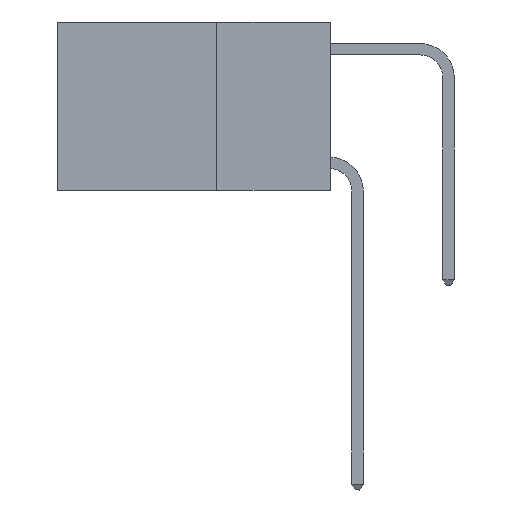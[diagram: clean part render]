
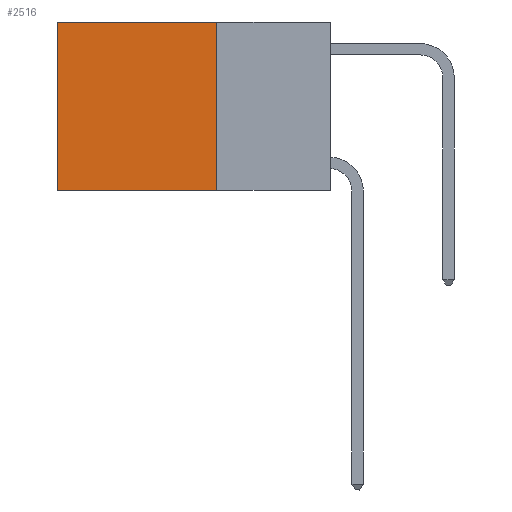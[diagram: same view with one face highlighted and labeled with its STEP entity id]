
A CAD part, left-side view. The second image highlights one B-rep face of the part: STEP entity #2516.
In plain terms, the highlighted planar face has unit normal (-1, 0, 0).
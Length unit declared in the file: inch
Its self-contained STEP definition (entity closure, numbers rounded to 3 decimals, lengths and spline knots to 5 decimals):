
#1464 = VECTOR ( 'NONE', #6346, 39.37008 ) ;
#2185 = ORIENTED_EDGE ( 'NONE', *, *, #26075, .F. ) ;
#2516 = ADVANCED_FACE ( 'NONE', ( #10999 ), #21430, .F. ) ;
#2658 = CARTESIAN_POINT ( 'NONE',  ( 0.2625, 0.25, 0. ) ) ;
#2849 = VERTEX_POINT ( 'NONE', #7916 ) ;
#4183 = LINE ( 'NONE', #4329, #1464 ) ;
#4329 = CARTESIAN_POINT ( 'NONE',  ( 0.2625, 0.25, -0.37 ) ) ;
#4627 = DIRECTION ( 'NONE',  ( 0., 0., -1. ) ) ;
#6046 = DIRECTION ( 'NONE',  ( 1., 0., 0. ) ) ;
#6346 = DIRECTION ( 'NONE',  ( 0., 1., 0. ) ) ;
#7273 = DIRECTION ( 'NONE',  ( 0., 0., -1. ) ) ;
#7916 = CARTESIAN_POINT ( 'NONE',  ( 0.2625, 0.6, -0.37 ) ) ;
#8099 = DIRECTION ( 'NONE',  ( 0., 0., -1. ) ) ;
#9724 = CARTESIAN_POINT ( 'NONE',  ( 0.2625, 0.6, 0. ) ) ;
#10724 = LINE ( 'NONE', #15518, #16401 ) ;
#10946 = CARTESIAN_POINT ( 'NONE',  ( 0.2625, 0.25, 0. ) ) ;
#10999 = FACE_OUTER_BOUND ( 'NONE', #18602, .T. ) ;
#11316 = ORIENTED_EDGE ( 'NONE', *, *, #17444, .T. ) ;
#15248 = ORIENTED_EDGE ( 'NONE', *, *, #21425, .F. ) ;
#15518 = CARTESIAN_POINT ( 'NONE',  ( 0.2625, 0.25, 0. ) ) ;
#16019 = EDGE_CURVE ( 'NONE', #23836, #22442, #22501, .T. ) ;
#16401 = VECTOR ( 'NONE', #4627, 39.37008 ) ;
#17006 = AXIS2_PLACEMENT_3D ( 'NONE', #19843, #6046, #8099 ) ;
#17444 = EDGE_CURVE ( 'NONE', #22442, #2849, #25091, .T. ) ;
#18409 = ORIENTED_EDGE ( 'NONE', *, *, #16019, .T. ) ;
#18602 = EDGE_LOOP ( 'NONE', ( #11316, #15248, #2185, #18409 ) ) ;
#18918 = VERTEX_POINT ( 'NONE', #27171 ) ;
#19843 = CARTESIAN_POINT ( 'NONE',  ( 0.2625, 0.25, 0. ) ) ;
#20331 = DIRECTION ( 'NONE',  ( 0., 1., 0. ) ) ;
#21425 = EDGE_CURVE ( 'NONE', #18918, #2849, #4183, .T. ) ;
#21430 = PLANE ( 'NONE',  #17006 ) ;
#22442 = VERTEX_POINT ( 'NONE', #22760 ) ;
#22501 = LINE ( 'NONE', #2658, #28008 ) ;
#22760 = CARTESIAN_POINT ( 'NONE',  ( 0.2625, 0.6, 0. ) ) ;
#23836 = VERTEX_POINT ( 'NONE', #10946 ) ;
#24810 = VECTOR ( 'NONE', #7273, 39.37008 ) ;
#25091 = LINE ( 'NONE', #9724, #24810 ) ;
#26075 = EDGE_CURVE ( 'NONE', #23836, #18918, #10724, .T. ) ;
#27171 = CARTESIAN_POINT ( 'NONE',  ( 0.2625, 0.25, -0.37 ) ) ;
#28008 = VECTOR ( 'NONE', #20331, 39.37008 ) ;
